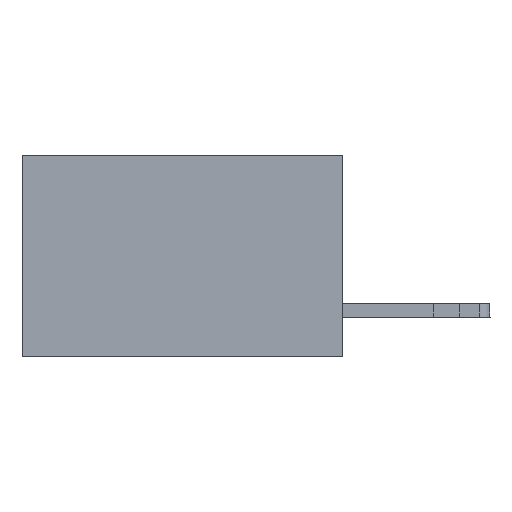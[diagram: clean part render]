
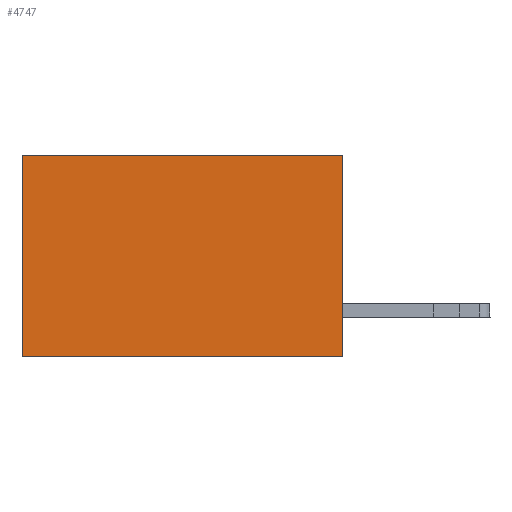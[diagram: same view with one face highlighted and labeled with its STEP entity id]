
A CAD part, left-side view. The second image highlights one B-rep face of the part: STEP entity #4747.
In plain terms, the highlighted planar face has unit normal (-1, 0, 0).
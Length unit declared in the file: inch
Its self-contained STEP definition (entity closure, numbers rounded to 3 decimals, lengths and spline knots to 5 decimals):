
#546 = CARTESIAN_POINT ( 'NONE',  ( 0.277, 0., -0.37 ) ) ;
#1347 = ORIENTED_EDGE ( 'NONE', *, *, #14618, .F. ) ;
#2350 = LINE ( 'NONE', #4195, #14642 ) ;
#3054 = CARTESIAN_POINT ( 'NONE',  ( 0.277, 0., 0. ) ) ;
#3270 = EDGE_CURVE ( 'NONE', #10853, #14440, #2350, .T. ) ;
#3677 = DIRECTION ( 'NONE',  ( 0., 1., 0. ) ) ;
#4195 = CARTESIAN_POINT ( 'NONE',  ( 0.277, 0., 0. ) ) ;
#4747 = ADVANCED_FACE ( 'NONE', ( #13620 ), #17060, .F. ) ;
#5048 = ORIENTED_EDGE ( 'NONE', *, *, #19387, .T. ) ;
#5907 = VECTOR ( 'NONE', #3677, 39.37008 ) ;
#6426 = EDGE_LOOP ( 'NONE', ( #5048, #1347, #18357, #11520 ) ) ;
#6721 = DIRECTION ( 'NONE',  ( 0., 0., -1. ) ) ;
#7533 = DIRECTION ( 'NONE',  ( 0., 1., 0. ) ) ;
#9290 = LINE ( 'NONE', #11578, #14370 ) ;
#9318 = LINE ( 'NONE', #546, #5907 ) ;
#10853 = VERTEX_POINT ( 'NONE', #3054 ) ;
#11028 = LINE ( 'NONE', #21721, #13698 ) ;
#11520 = ORIENTED_EDGE ( 'NONE', *, *, #3270, .T. ) ;
#11565 = CARTESIAN_POINT ( 'NONE',  ( 0.277, 0., -0.37 ) ) ;
#11578 = CARTESIAN_POINT ( 'NONE',  ( 0.277, 0., -0.37 ) ) ;
#13620 = FACE_OUTER_BOUND ( 'NONE', #6426, .T. ) ;
#13698 = VECTOR ( 'NONE', #16522, 39.37008 ) ;
#14370 = VECTOR ( 'NONE', #20000, 39.37008 ) ;
#14440 = VERTEX_POINT ( 'NONE', #21078 ) ;
#14618 = EDGE_CURVE ( 'NONE', #15800, #21440, #9318, .T. ) ;
#14642 = VECTOR ( 'NONE', #7533, 39.37008 ) ;
#15800 = VERTEX_POINT ( 'NONE', #18211 ) ;
#16522 = DIRECTION ( 'NONE',  ( 0., 0., -1. ) ) ;
#16644 = EDGE_CURVE ( 'NONE', #10853, #15800, #9290, .T. ) ;
#17060 = PLANE ( 'NONE',  #18101 ) ;
#17401 = CARTESIAN_POINT ( 'NONE',  ( 0.277, 0.59, -0.37 ) ) ;
#18101 = AXIS2_PLACEMENT_3D ( 'NONE', #11565, #22512, #6721 ) ;
#18211 = CARTESIAN_POINT ( 'NONE',  ( 0.277, 0., -0.37 ) ) ;
#18357 = ORIENTED_EDGE ( 'NONE', *, *, #16644, .F. ) ;
#19387 = EDGE_CURVE ( 'NONE', #14440, #21440, #11028, .T. ) ;
#20000 = DIRECTION ( 'NONE',  ( 0., 0., -1. ) ) ;
#21078 = CARTESIAN_POINT ( 'NONE',  ( 0.277, 0.59, 0. ) ) ;
#21440 = VERTEX_POINT ( 'NONE', #17401 ) ;
#21721 = CARTESIAN_POINT ( 'NONE',  ( 0.277, 0.59, -0.37 ) ) ;
#22512 = DIRECTION ( 'NONE',  ( 1., 0., 0. ) ) ;
